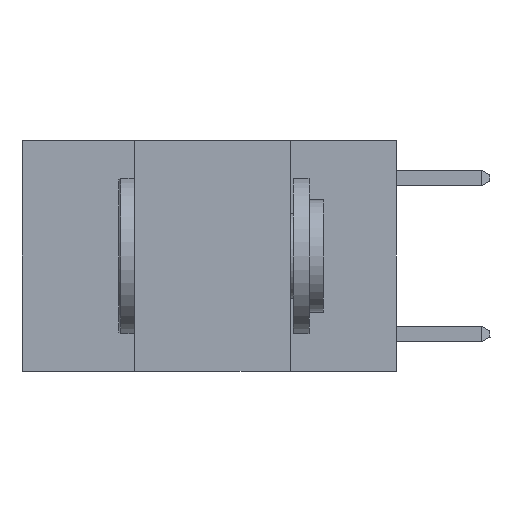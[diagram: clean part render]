
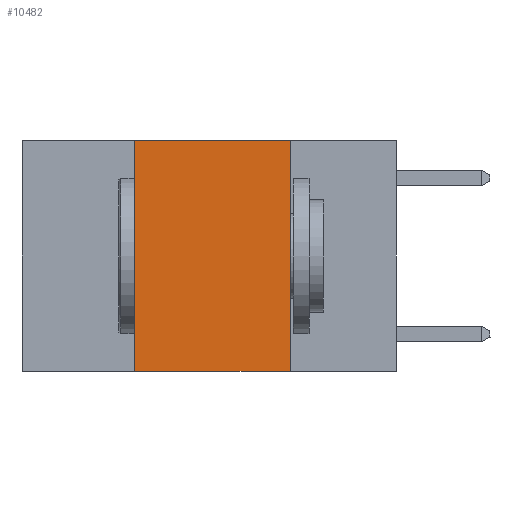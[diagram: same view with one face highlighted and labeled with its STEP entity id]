
A CAD part, left-side view. The second image highlights one B-rep face of the part: STEP entity #10482.
In plain terms, the highlighted planar face has unit normal (-1, 0, 0).
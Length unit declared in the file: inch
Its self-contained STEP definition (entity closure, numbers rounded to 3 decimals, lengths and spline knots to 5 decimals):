
#363 = VERTEX_POINT ( 'NONE', #22035 ) ;
#797 = VERTEX_POINT ( 'NONE', #20482 ) ;
#2546 = DIRECTION ( 'NONE',  ( 0., 0., 1. ) ) ;
#2797 = AXIS2_PLACEMENT_3D ( 'NONE', #15795, #17983, #4881 ) ;
#3343 = CARTESIAN_POINT ( 'NONE',  ( 0., 0.17, 0. ) ) ;
#3922 = DIRECTION ( 'NONE',  ( 0., -1., 0. ) ) ;
#4881 = DIRECTION ( 'NONE',  ( 0., 0., -1. ) ) ;
#5249 = LINE ( 'NONE', #6913, #16192 ) ;
#6349 = VECTOR ( 'NONE', #3922, 39.37008 ) ;
#6718 = ORIENTED_EDGE ( 'NONE', *, *, #26883, .F. ) ;
#6913 = CARTESIAN_POINT ( 'NONE',  ( 0., 0.17, 0. ) ) ;
#8307 = CARTESIAN_POINT ( 'NONE',  ( 0., 0.6, -0.37 ) ) ;
#9048 = VECTOR ( 'NONE', #2546, 39.37008 ) ;
#9307 = VERTEX_POINT ( 'NONE', #18206 ) ;
#10455 = EDGE_CURVE ( 'NONE', #797, #9307, #20643, .T. ) ;
#10482 = ADVANCED_FACE ( 'NONE', ( #13469 ), #20057, .F. ) ;
#11174 = ORIENTED_EDGE ( 'NONE', *, *, #17565, .F. ) ;
#11249 = DIRECTION ( 'NONE',  ( 0., 0., -1. ) ) ;
#12462 = EDGE_LOOP ( 'NONE', ( #6718, #11174, #12584, #13025 ) ) ;
#12584 = ORIENTED_EDGE ( 'NONE', *, *, #10455, .F. ) ;
#12799 = LINE ( 'NONE', #17034, #6349 ) ;
#13025 = ORIENTED_EDGE ( 'NONE', *, *, #15383, .T. ) ;
#13469 = FACE_OUTER_BOUND ( 'NONE', #12462, .T. ) ;
#15383 = EDGE_CURVE ( 'NONE', #797, #363, #27411, .T. ) ;
#15795 = CARTESIAN_POINT ( 'NONE',  ( 0., 0.6, 0. ) ) ;
#16192 = VECTOR ( 'NONE', #11249, 39.37008 ) ;
#17034 = CARTESIAN_POINT ( 'NONE',  ( 0., 0.6, 0. ) ) ;
#17391 = VERTEX_POINT ( 'NONE', #3343 ) ;
#17565 = EDGE_CURVE ( 'NONE', #9307, #17391, #12799, .T. ) ;
#17888 = CARTESIAN_POINT ( 'NONE',  ( 0., 0.42, 0. ) ) ;
#17983 = DIRECTION ( 'NONE',  ( 1., 0., 0. ) ) ;
#18206 = CARTESIAN_POINT ( 'NONE',  ( 0., 0.42, 0. ) ) ;
#20057 = PLANE ( 'NONE',  #2797 ) ;
#20482 = CARTESIAN_POINT ( 'NONE',  ( 0., 0.42, -0.37 ) ) ;
#20643 = LINE ( 'NONE', #17888, #9048 ) ;
#21140 = VECTOR ( 'NONE', #25598, 39.37008 ) ;
#22035 = CARTESIAN_POINT ( 'NONE',  ( 0., 0.17, -0.37 ) ) ;
#25598 = DIRECTION ( 'NONE',  ( 0., -1., 0. ) ) ;
#26883 = EDGE_CURVE ( 'NONE', #17391, #363, #5249, .T. ) ;
#27411 = LINE ( 'NONE', #8307, #21140 ) ;
